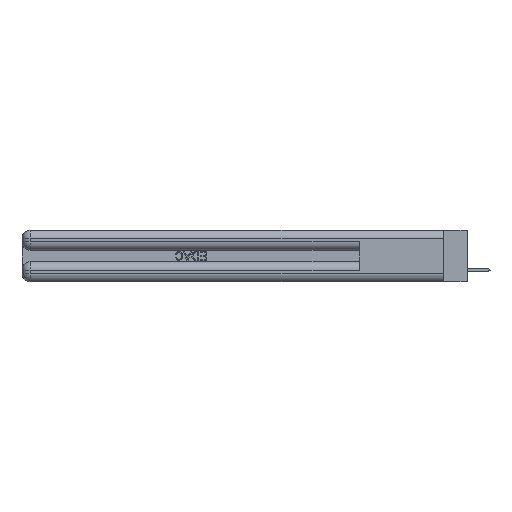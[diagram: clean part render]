
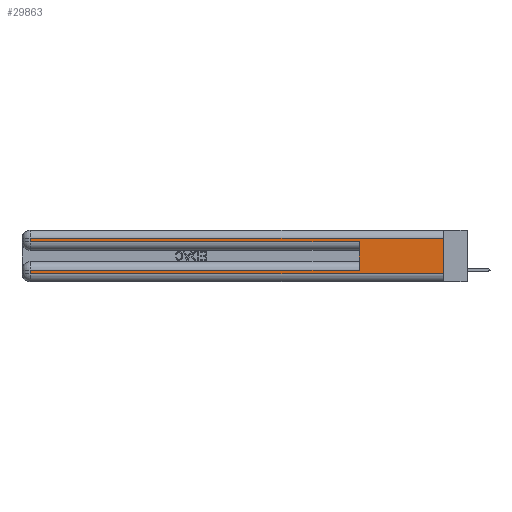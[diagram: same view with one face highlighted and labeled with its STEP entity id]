
A CAD part, left-side view. The second image highlights one B-rep face of the part: STEP entity #29863.
In plain terms, the highlighted planar face has unit normal (-1, 0, 0).
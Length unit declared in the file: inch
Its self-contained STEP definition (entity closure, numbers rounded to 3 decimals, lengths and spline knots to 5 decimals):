
#335 = VECTOR ( 'NONE', #4270, 39.37008 ) ;
#1662 = DIRECTION ( 'NONE',  ( 0., 1., 0. ) ) ;
#1828 = ORIENTED_EDGE ( 'NONE', *, *, #8527, .T. ) ;
#2551 = DIRECTION ( 'NONE',  ( 0., -1., 0. ) ) ;
#2736 = EDGE_CURVE ( 'NONE', #11592, #15279, #40446, .T. ) ;
#3420 = CARTESIAN_POINT ( 'NONE',  ( 0., 0., 0.285 ) ) ;
#4244 = VECTOR ( 'NONE', #9057, 39.37008 ) ;
#4270 = DIRECTION ( 'NONE',  ( 0., -1., 0. ) ) ;
#4585 = CARTESIAN_POINT ( 'NONE',  ( 0., 2.94, 0.37 ) ) ;
#5858 = FACE_OUTER_BOUND ( 'NONE', #42886, .T. ) ;
#6233 = VERTEX_POINT ( 'NONE', #7592 ) ;
#7244 = DIRECTION ( 'NONE',  ( 0., 0., 1. ) ) ;
#7276 = ORIENTED_EDGE ( 'NONE', *, *, #37593, .T. ) ;
#7592 = CARTESIAN_POINT ( 'NONE',  ( 0., 2.94, 0.06 ) ) ;
#8527 = EDGE_CURVE ( 'NONE', #36912, #6233, #9509, .T. ) ;
#9019 = VECTOR ( 'NONE', #7244, 39.37008 ) ;
#9057 = DIRECTION ( 'NONE',  ( 0., 0., -1. ) ) ;
#9384 = VERTEX_POINT ( 'NONE', #39461 ) ;
#9505 = LINE ( 'NONE', #31640, #4244 ) ;
#9509 = LINE ( 'NONE', #4585, #36807 ) ;
#10078 = CARTESIAN_POINT ( 'NONE',  ( 0., 0.6, 0.285 ) ) ;
#10292 = DIRECTION ( 'NONE',  ( 0., 0., -1. ) ) ;
#10691 = CARTESIAN_POINT ( 'NONE',  ( 0., 0.6, 0.145 ) ) ;
#11287 = ORIENTED_EDGE ( 'NONE', *, *, #19418, .F. ) ;
#11592 = VERTEX_POINT ( 'NONE', #32885 ) ;
#12123 = CARTESIAN_POINT ( 'NONE',  ( 0., 0., 0.085 ) ) ;
#12268 = EDGE_CURVE ( 'NONE', #22915, #27053, #28844, .T. ) ;
#12608 = LINE ( 'NONE', #29843, #335 ) ;
#13562 = DIRECTION ( 'NONE',  ( 0., 0., -1. ) ) ;
#13815 = LINE ( 'NONE', #12123, #37051 ) ;
#14610 = LINE ( 'NONE', #24591, #42353 ) ;
#15279 = VERTEX_POINT ( 'NONE', #37422 ) ;
#16829 = EDGE_CURVE ( 'NONE', #15279, #9384, #9505, .T. ) ;
#17151 = CARTESIAN_POINT ( 'NONE',  ( 0., 0., 0.31 ) ) ;
#18806 = VERTEX_POINT ( 'NONE', #33185 ) ;
#19418 = EDGE_CURVE ( 'NONE', #11592, #18806, #14610, .T. ) ;
#20809 = ORIENTED_EDGE ( 'NONE', *, *, #2736, .T. ) ;
#21098 = EDGE_CURVE ( 'NONE', #9384, #27053, #21949, .T. ) ;
#21949 = LINE ( 'NONE', #3420, #45116 ) ;
#22262 = CARTESIAN_POINT ( 'NONE',  ( 0., 2.94, 0.085 ) ) ;
#22915 = VERTEX_POINT ( 'NONE', #25595 ) ;
#24591 = CARTESIAN_POINT ( 'NONE',  ( 0., 0., 0.37 ) ) ;
#25455 = AXIS2_PLACEMENT_3D ( 'NONE', #32886, #40159, #47628 ) ;
#25595 = CARTESIAN_POINT ( 'NONE',  ( 0., 0.6, 0.085 ) ) ;
#25634 = ORIENTED_EDGE ( 'NONE', *, *, #45130, .T. ) ;
#26597 = ORIENTED_EDGE ( 'NONE', *, *, #21098, .T. ) ;
#27053 = VERTEX_POINT ( 'NONE', #10078 ) ;
#27087 = DIRECTION ( 'NONE',  ( 0., 1., 0. ) ) ;
#28844 = LINE ( 'NONE', #10691, #9019 ) ;
#29687 = ORIENTED_EDGE ( 'NONE', *, *, #12268, .F. ) ;
#29843 = CARTESIAN_POINT ( 'NONE',  ( 0., 0., 0.06 ) ) ;
#29863 = ADVANCED_FACE ( 'NONE', ( #5858 ), #46983, .F. ) ;
#31640 = CARTESIAN_POINT ( 'NONE',  ( 0., 2.94, 0.37 ) ) ;
#32885 = CARTESIAN_POINT ( 'NONE',  ( 0., 0., 0.31 ) ) ;
#32886 = CARTESIAN_POINT ( 'NONE',  ( 0., 0., 0.37 ) ) ;
#33185 = CARTESIAN_POINT ( 'NONE',  ( 0., 0., 0.06 ) ) ;
#36807 = VECTOR ( 'NONE', #10292, 39.37008 ) ;
#36912 = VERTEX_POINT ( 'NONE', #22262 ) ;
#37051 = VECTOR ( 'NONE', #27087, 39.37008 ) ;
#37422 = CARTESIAN_POINT ( 'NONE',  ( 0., 2.94, 0.31 ) ) ;
#37593 = EDGE_CURVE ( 'NONE', #6233, #18806, #12608, .T. ) ;
#39262 = VECTOR ( 'NONE', #1662, 39.37008 ) ;
#39461 = CARTESIAN_POINT ( 'NONE',  ( 0., 2.94, 0.285 ) ) ;
#40159 = DIRECTION ( 'NONE',  ( 1., 0., 0. ) ) ;
#40446 = LINE ( 'NONE', #17151, #39262 ) ;
#42353 = VECTOR ( 'NONE', #13562, 39.37008 ) ;
#42886 = EDGE_LOOP ( 'NONE', ( #11287, #20809, #43253, #26597, #29687, #25634, #1828, #7276 ) ) ;
#43253 = ORIENTED_EDGE ( 'NONE', *, *, #16829, .T. ) ;
#45116 = VECTOR ( 'NONE', #2551, 39.37008 ) ;
#45130 = EDGE_CURVE ( 'NONE', #22915, #36912, #13815, .T. ) ;
#46983 = PLANE ( 'NONE',  #25455 ) ;
#47628 = DIRECTION ( 'NONE',  ( 0., 0., -1. ) ) ;
